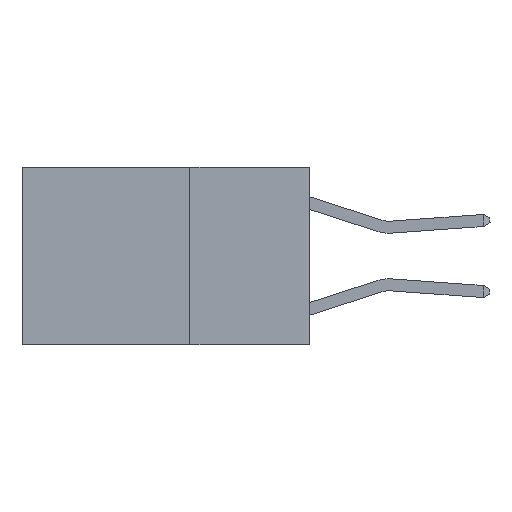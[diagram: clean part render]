
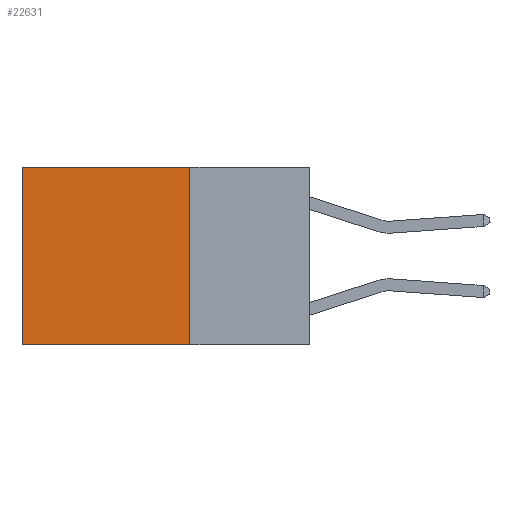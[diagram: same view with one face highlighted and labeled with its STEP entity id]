
A CAD part, left-side view. The second image highlights one B-rep face of the part: STEP entity #22631.
In plain terms, the highlighted planar face has unit normal (-1, 0, 0).
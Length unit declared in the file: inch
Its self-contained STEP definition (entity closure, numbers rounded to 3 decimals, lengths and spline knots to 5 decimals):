
#202 = EDGE_LOOP ( 'NONE', ( #27333, #25686, #7705, #24189 ) ) ;
#533 = EDGE_CURVE ( 'NONE', #7869, #2271, #23834, .T. ) ;
#1756 = LINE ( 'NONE', #11506, #5015 ) ;
#2271 = VERTEX_POINT ( 'NONE', #13405 ) ;
#2983 = VECTOR ( 'NONE', #26343, 39.37008 ) ;
#4047 = FACE_OUTER_BOUND ( 'NONE', #202, .T. ) ;
#4741 = DIRECTION ( 'NONE',  ( 0., 0., -1. ) ) ;
#5015 = VECTOR ( 'NONE', #18455, 39.37008 ) ;
#6945 = LINE ( 'NONE', #7585, #22983 ) ;
#7571 = EDGE_CURVE ( 'NONE', #14511, #26460, #6945, .T. ) ;
#7585 = CARTESIAN_POINT ( 'NONE',  ( 0.2625, 0.6, 0. ) ) ;
#7705 = ORIENTED_EDGE ( 'NONE', *, *, #533, .F. ) ;
#7869 = VERTEX_POINT ( 'NONE', #30763 ) ;
#8620 = DIRECTION ( 'NONE',  ( 1., 0., 0. ) ) ;
#9278 = AXIS2_PLACEMENT_3D ( 'NONE', #11439, #8620, #21200 ) ;
#9975 = LINE ( 'NONE', #26798, #13997 ) ;
#10613 = CARTESIAN_POINT ( 'NONE',  ( 0.2625, 0.6, 0. ) ) ;
#11439 = CARTESIAN_POINT ( 'NONE',  ( 0.2625, 0.25, 0. ) ) ;
#11506 = CARTESIAN_POINT ( 'NONE',  ( 0.2625, 0.25, -0.37 ) ) ;
#13405 = CARTESIAN_POINT ( 'NONE',  ( 0.2625, 0.25, -0.37 ) ) ;
#13997 = VECTOR ( 'NONE', #29310, 39.37008 ) ;
#14511 = VERTEX_POINT ( 'NONE', #10613 ) ;
#18455 = DIRECTION ( 'NONE',  ( 0., 1., 0. ) ) ;
#21200 = DIRECTION ( 'NONE',  ( 0., 0., -1. ) ) ;
#21497 = CARTESIAN_POINT ( 'NONE',  ( 0.2625, 0.25, 0. ) ) ;
#22631 = ADVANCED_FACE ( 'NONE', ( #4047 ), #30610, .F. ) ;
#22983 = VECTOR ( 'NONE', #4741, 39.37008 ) ;
#23834 = LINE ( 'NONE', #21497, #2983 ) ;
#24189 = ORIENTED_EDGE ( 'NONE', *, *, #28081, .T. ) ;
#25686 = ORIENTED_EDGE ( 'NONE', *, *, #29820, .F. ) ;
#26343 = DIRECTION ( 'NONE',  ( 0., 0., -1. ) ) ;
#26460 = VERTEX_POINT ( 'NONE', #27678 ) ;
#26798 = CARTESIAN_POINT ( 'NONE',  ( 0.2625, 0.25, 0. ) ) ;
#27333 = ORIENTED_EDGE ( 'NONE', *, *, #7571, .T. ) ;
#27678 = CARTESIAN_POINT ( 'NONE',  ( 0.2625, 0.6, -0.37 ) ) ;
#28081 = EDGE_CURVE ( 'NONE', #7869, #14511, #9975, .T. ) ;
#29310 = DIRECTION ( 'NONE',  ( 0., 1., 0. ) ) ;
#29820 = EDGE_CURVE ( 'NONE', #2271, #26460, #1756, .T. ) ;
#30610 = PLANE ( 'NONE',  #9278 ) ;
#30763 = CARTESIAN_POINT ( 'NONE',  ( 0.2625, 0.25, 0. ) ) ;
